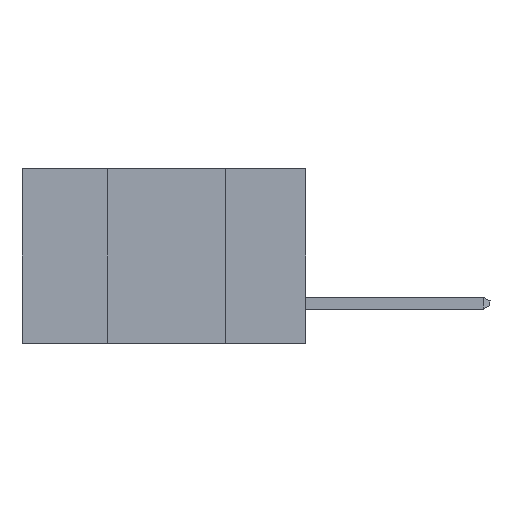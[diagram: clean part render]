
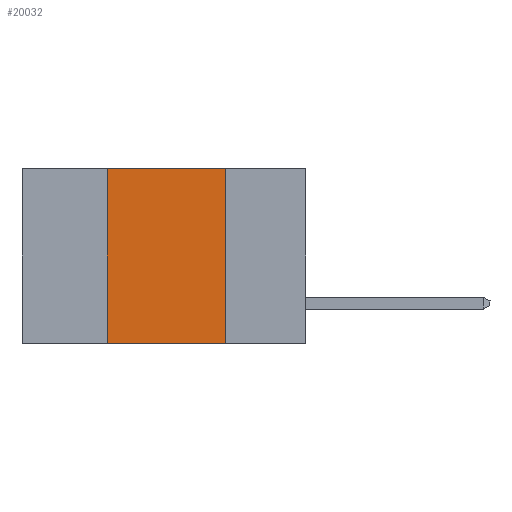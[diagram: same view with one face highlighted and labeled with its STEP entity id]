
A CAD part, left-side view. The second image highlights one B-rep face of the part: STEP entity #20032.
In plain terms, the highlighted planar face has unit normal (-1, 0, 0).
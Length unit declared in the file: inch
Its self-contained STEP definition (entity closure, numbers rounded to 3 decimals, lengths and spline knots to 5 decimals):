
#576 = VECTOR ( 'NONE', #5293, 39.37008 ) ;
#1223 = LINE ( 'NONE', #5478, #576 ) ;
#1519 = VERTEX_POINT ( 'NONE', #12735 ) ;
#1948 = DIRECTION ( 'NONE',  ( 0., 0., -1. ) ) ;
#3761 = EDGE_CURVE ( 'NONE', #22359, #1519, #24434, .T. ) ;
#4913 = CARTESIAN_POINT ( 'NONE',  ( 0., 0.42, 0. ) ) ;
#5293 = DIRECTION ( 'NONE',  ( 0., -1., 0. ) ) ;
#5478 = CARTESIAN_POINT ( 'NONE',  ( 0., 0.6, -0.37 ) ) ;
#6950 = ORIENTED_EDGE ( 'NONE', *, *, #20662, .F. ) ;
#7551 = ORIENTED_EDGE ( 'NONE', *, *, #3761, .F. ) ;
#8371 = CARTESIAN_POINT ( 'NONE',  ( 0., 0.17, -0.37 ) ) ;
#9646 = AXIS2_PLACEMENT_3D ( 'NONE', #24598, #13618, #1948 ) ;
#11126 = EDGE_CURVE ( 'NONE', #20411, #16580, #1223, .T. ) ;
#11330 = CARTESIAN_POINT ( 'NONE',  ( 0., 0.42, -0.37 ) ) ;
#11689 = PLANE ( 'NONE',  #9646 ) ;
#12735 = CARTESIAN_POINT ( 'NONE',  ( 0., 0.17, 0. ) ) ;
#13618 = DIRECTION ( 'NONE',  ( 1., 0., 0. ) ) ;
#14393 = EDGE_LOOP ( 'NONE', ( #22584, #7551, #6950, #21433 ) ) ;
#15291 = VECTOR ( 'NONE', #23233, 39.37008 ) ;
#16376 = VECTOR ( 'NONE', #20844, 39.37008 ) ;
#16580 = VERTEX_POINT ( 'NONE', #18783 ) ;
#17144 = CARTESIAN_POINT ( 'NONE',  ( 0., 0.42, -0.37 ) ) ;
#18783 = CARTESIAN_POINT ( 'NONE',  ( 0., 0.17, -0.37 ) ) ;
#20032 = ADVANCED_FACE ( 'NONE', ( #22164 ), #11689, .F. ) ;
#20053 = VECTOR ( 'NONE', #21527, 39.37008 ) ;
#20411 = VERTEX_POINT ( 'NONE', #11330 ) ;
#20662 = EDGE_CURVE ( 'NONE', #20411, #22359, #21262, .T. ) ;
#20844 = DIRECTION ( 'NONE',  ( 0., 0., 1. ) ) ;
#21262 = LINE ( 'NONE', #17144, #16376 ) ;
#21433 = ORIENTED_EDGE ( 'NONE', *, *, #11126, .T. ) ;
#21527 = DIRECTION ( 'NONE',  ( 0., 0., -1. ) ) ;
#21593 = EDGE_CURVE ( 'NONE', #1519, #16580, #24312, .T. ) ;
#22164 = FACE_OUTER_BOUND ( 'NONE', #14393, .T. ) ;
#22359 = VERTEX_POINT ( 'NONE', #4913 ) ;
#22584 = ORIENTED_EDGE ( 'NONE', *, *, #21593, .F. ) ;
#23233 = DIRECTION ( 'NONE',  ( 0., -1., 0. ) ) ;
#24048 = CARTESIAN_POINT ( 'NONE',  ( 0., 0.6, 0. ) ) ;
#24312 = LINE ( 'NONE', #8371, #20053 ) ;
#24434 = LINE ( 'NONE', #24048, #15291 ) ;
#24598 = CARTESIAN_POINT ( 'NONE',  ( 0., 0.6, 0. ) ) ;
